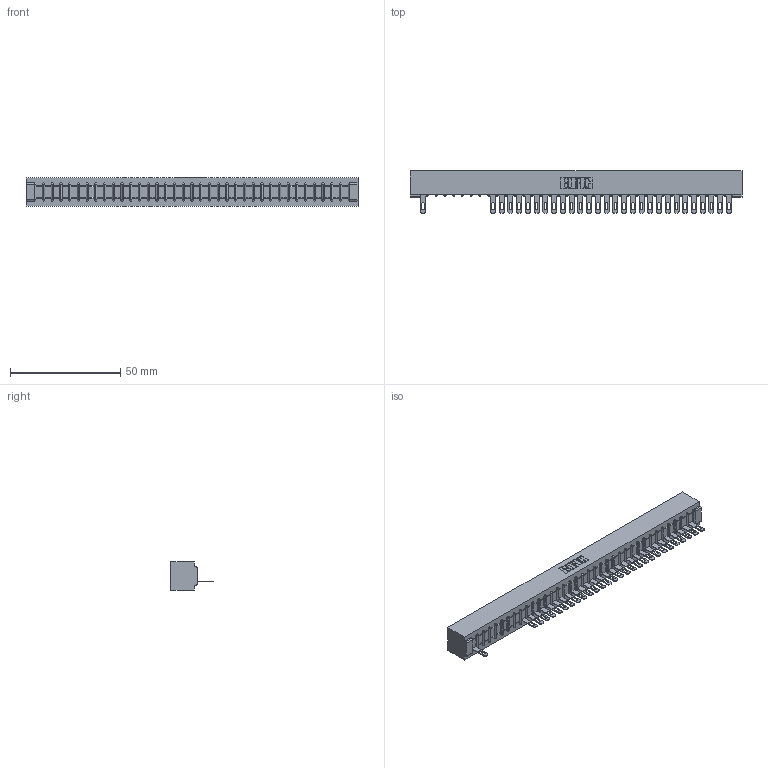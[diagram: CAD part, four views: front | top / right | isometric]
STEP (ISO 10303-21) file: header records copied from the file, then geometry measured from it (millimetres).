
FILE_DESCRIPTION (( 'STEP AP203' ), '1' );
FILE_NAME ('307-036-505-101.STEP', '2018-08-05T07:45:16', ( '' ), ( '' ), 'SwSTEP 2.0', 'SolidWorks 2016', '' );
FILE_SCHEMA (( 'CONFIG_CONTROL_DESIGN' ));
Length unit declared in the file: inch
Products named in the file (3): 307 Part_No Mounting Lugs; 307-290-001_505; 307-036-505-101
Assembly tree (30 placements, depth 2):
  307-036-505-101
    307 Part_No Mounting Lugs
    307-290-001_505  x29
Bounding box: 150.52 x 19.18 x 12.7 mm (x, y, z)
Volume: 16038.8 mm3; surface area: 16633.1 mm2
Topology: 30 solids, 30 shells, 1911 faces, 5445 edges, 3490 vertices
Faces by surface type: plane 1194, cylinder 643, sphere 74
Entity records: 31074 total; most frequent: CARTESIAN_POINT 5261, ORIENTED_EDGE 5254, DIRECTION 5113, EDGE_CURVE 2627, VECTOR 2013, LINE 2013, VERTEX_POINT 1698, AXIS2_PLACEMENT_3D 1550
